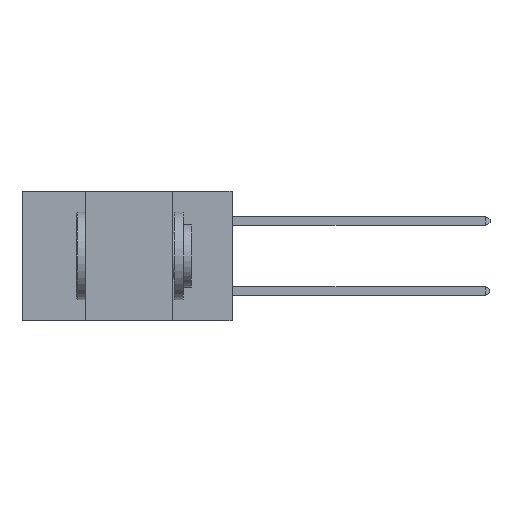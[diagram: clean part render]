
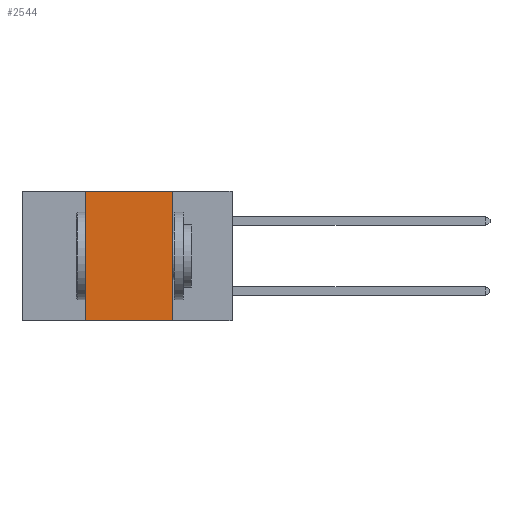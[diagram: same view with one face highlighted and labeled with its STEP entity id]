
A CAD part, left-side view. The second image highlights one B-rep face of the part: STEP entity #2544.
In plain terms, the highlighted planar face has unit normal (-1, 0, 0).
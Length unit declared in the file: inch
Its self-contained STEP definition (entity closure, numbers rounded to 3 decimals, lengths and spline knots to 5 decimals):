
#20 = VERTEX_POINT ( 'NONE', #802 ) ;
#42 = FACE_OUTER_BOUND ( 'NONE', #12329, .T. ) ;
#438 = EDGE_CURVE ( 'NONE', #5546, #6278, #9879, .T. ) ;
#477 = EDGE_CURVE ( 'NONE', #5546, #20, #7028, .T. ) ;
#721 = ORIENTED_EDGE ( 'NONE', *, *, #9044, .F. ) ;
#802 = CARTESIAN_POINT ( 'NONE',  ( 0., 0.17, -0.37 ) ) ;
#825 = DIRECTION ( 'NONE',  ( 0., -1., 0. ) ) ;
#883 = CARTESIAN_POINT ( 'NONE',  ( 0., 0.6, -0.37 ) ) ;
#2283 = VECTOR ( 'NONE', #4555, 39.37008 ) ;
#2544 = ADVANCED_FACE ( 'NONE', ( #42 ), #3906, .F. ) ;
#3610 = DIRECTION ( 'NONE',  ( 0., 0., -1. ) ) ;
#3661 = DIRECTION ( 'NONE',  ( 1., 0., 0. ) ) ;
#3706 = CARTESIAN_POINT ( 'NONE',  ( 0., 0.6, 0. ) ) ;
#3906 = PLANE ( 'NONE',  #11163 ) ;
#4555 = DIRECTION ( 'NONE',  ( 0., 0., 1. ) ) ;
#4722 = CARTESIAN_POINT ( 'NONE',  ( 0., 0.6, 0. ) ) ;
#4803 = CARTESIAN_POINT ( 'NONE',  ( 0., 0.42, 0. ) ) ;
#5017 = EDGE_CURVE ( 'NONE', #10321, #20, #6864, .T. ) ;
#5546 = VERTEX_POINT ( 'NONE', #8265 ) ;
#5736 = DIRECTION ( 'NONE',  ( 0., -1., 0. ) ) ;
#6278 = VERTEX_POINT ( 'NONE', #4803 ) ;
#6588 = VECTOR ( 'NONE', #11208, 39.37008 ) ;
#6864 = LINE ( 'NONE', #11342, #6588 ) ;
#6964 = LINE ( 'NONE', #4722, #11641 ) ;
#7028 = LINE ( 'NONE', #883, #11700 ) ;
#7789 = ORIENTED_EDGE ( 'NONE', *, *, #5017, .F. ) ;
#7899 = CARTESIAN_POINT ( 'NONE',  ( 0., 0.42, 0. ) ) ;
#8265 = CARTESIAN_POINT ( 'NONE',  ( 0., 0.42, -0.37 ) ) ;
#9044 = EDGE_CURVE ( 'NONE', #6278, #10321, #6964, .T. ) ;
#9879 = LINE ( 'NONE', #7899, #2283 ) ;
#9934 = CARTESIAN_POINT ( 'NONE',  ( 0., 0.17, 0. ) ) ;
#10321 = VERTEX_POINT ( 'NONE', #9934 ) ;
#11082 = ORIENTED_EDGE ( 'NONE', *, *, #477, .T. ) ;
#11163 = AXIS2_PLACEMENT_3D ( 'NONE', #3706, #3661, #3610 ) ;
#11208 = DIRECTION ( 'NONE',  ( 0., 0., -1. ) ) ;
#11342 = CARTESIAN_POINT ( 'NONE',  ( 0., 0.17, 0. ) ) ;
#11641 = VECTOR ( 'NONE', #5736, 39.37008 ) ;
#11676 = ORIENTED_EDGE ( 'NONE', *, *, #438, .F. ) ;
#11700 = VECTOR ( 'NONE', #825, 39.37008 ) ;
#12329 = EDGE_LOOP ( 'NONE', ( #7789, #721, #11676, #11082 ) ) ;
